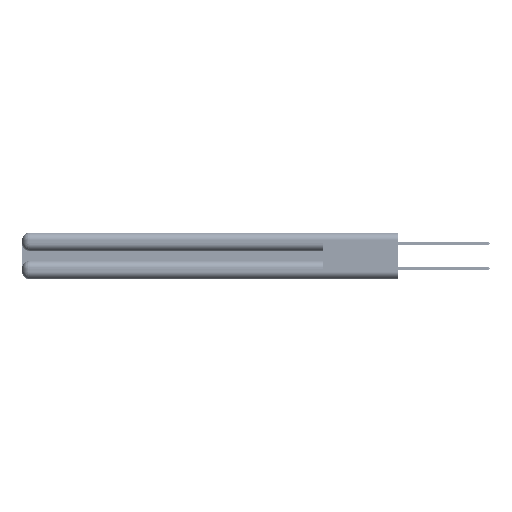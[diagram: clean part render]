
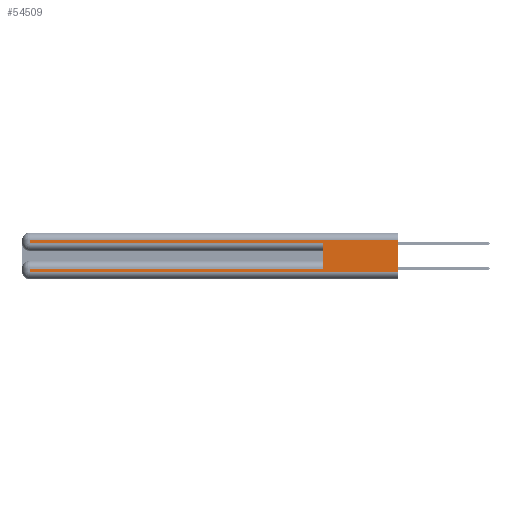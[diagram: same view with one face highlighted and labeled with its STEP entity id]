
A CAD part, left-side view. The second image highlights one B-rep face of the part: STEP entity #54509.
In plain terms, the highlighted planar face has unit normal (-1, 0, 0).
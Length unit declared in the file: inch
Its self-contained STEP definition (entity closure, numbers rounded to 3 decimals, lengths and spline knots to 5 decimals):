
#398 = VECTOR ( 'NONE', #5086, 39.37008 ) ;
#578 = VERTEX_POINT ( 'NONE', #2584 ) ;
#615 = CARTESIAN_POINT ( 'NONE',  ( 0., 0., 0.06 ) ) ;
#1155 = ORIENTED_EDGE ( 'NONE', *, *, #53234, .T. ) ;
#1574 = VECTOR ( 'NONE', #17906, 39.37008 ) ;
#2584 = CARTESIAN_POINT ( 'NONE',  ( 0., 0.6, 0.085 ) ) ;
#5034 = CARTESIAN_POINT ( 'NONE',  ( 0., 2.94, 0.37 ) ) ;
#5086 = DIRECTION ( 'NONE',  ( 0., 0., -1. ) ) ;
#5473 = VERTEX_POINT ( 'NONE', #21969 ) ;
#5600 = FACE_OUTER_BOUND ( 'NONE', #11197, .T. ) ;
#6402 = LINE ( 'NONE', #31272, #38980 ) ;
#7003 = ORIENTED_EDGE ( 'NONE', *, *, #23486, .F. ) ;
#7618 = CARTESIAN_POINT ( 'NONE',  ( 0., 0., 0.06 ) ) ;
#8330 = VECTOR ( 'NONE', #22632, 39.37008 ) ;
#8493 = CARTESIAN_POINT ( 'NONE',  ( 0., 0., 0.37 ) ) ;
#9296 = DIRECTION ( 'NONE',  ( 0., 0., -1. ) ) ;
#9761 = LINE ( 'NONE', #21096, #29712 ) ;
#10729 = CARTESIAN_POINT ( 'NONE',  ( 0., 2.94, 0.31 ) ) ;
#11197 = EDGE_LOOP ( 'NONE', ( #7003, #38644, #1155, #52044, #32829, #33176, #42025, #19998 ) ) ;
#12779 = DIRECTION ( 'NONE',  ( 0., 0., -1. ) ) ;
#12935 = VERTEX_POINT ( 'NONE', #10729 ) ;
#13240 = CARTESIAN_POINT ( 'NONE',  ( 0., 0.6, 0.285 ) ) ;
#14727 = VECTOR ( 'NONE', #20359, 39.37008 ) ;
#17906 = DIRECTION ( 'NONE',  ( 0., 0., 1. ) ) ;
#18385 = EDGE_CURVE ( 'NONE', #5473, #44259, #18519, .T. ) ;
#18519 = LINE ( 'NONE', #7618, #28480 ) ;
#19662 = LINE ( 'NONE', #52302, #8330 ) ;
#19998 = ORIENTED_EDGE ( 'NONE', *, *, #18385, .T. ) ;
#20359 = DIRECTION ( 'NONE',  ( 0., 0., -1. ) ) ;
#21096 = CARTESIAN_POINT ( 'NONE',  ( 0., 0., 0.285 ) ) ;
#21969 = CARTESIAN_POINT ( 'NONE',  ( 0., 2.94, 0.06 ) ) ;
#22632 = DIRECTION ( 'NONE',  ( 0., 1., 0. ) ) ;
#23486 = EDGE_CURVE ( 'NONE', #52811, #44259, #48574, .T. ) ;
#25427 = PLANE ( 'NONE',  #37599 ) ;
#26331 = EDGE_CURVE ( 'NONE', #32562, #36305, #9761, .T. ) ;
#27882 = EDGE_CURVE ( 'NONE', #52811, #12935, #19662, .T. ) ;
#28480 = VECTOR ( 'NONE', #37346, 39.37008 ) ;
#28507 = EDGE_CURVE ( 'NONE', #578, #36305, #35522, .T. ) ;
#29712 = VECTOR ( 'NONE', #46698, 39.37008 ) ;
#31272 = CARTESIAN_POINT ( 'NONE',  ( 0., 0., 0.085 ) ) ;
#31387 = VECTOR ( 'NONE', #9296, 39.37008 ) ;
#32481 = CARTESIAN_POINT ( 'NONE',  ( 0., 2.94, 0.285 ) ) ;
#32562 = VERTEX_POINT ( 'NONE', #32481 ) ;
#32829 = ORIENTED_EDGE ( 'NONE', *, *, #28507, .F. ) ;
#33176 = ORIENTED_EDGE ( 'NONE', *, *, #53359, .T. ) ;
#34354 = LINE ( 'NONE', #34819, #398 ) ;
#34819 = CARTESIAN_POINT ( 'NONE',  ( 0., 2.94, 0.37 ) ) ;
#35522 = LINE ( 'NONE', #47583, #1574 ) ;
#35553 = DIRECTION ( 'NONE',  ( 0., 1., 0. ) ) ;
#35851 = VERTEX_POINT ( 'NONE', #52831 ) ;
#36305 = VERTEX_POINT ( 'NONE', #13240 ) ;
#37346 = DIRECTION ( 'NONE',  ( 0., -1., 0. ) ) ;
#37599 = AXIS2_PLACEMENT_3D ( 'NONE', #8493, #38223, #12779 ) ;
#38223 = DIRECTION ( 'NONE',  ( 1., 0., 0. ) ) ;
#38644 = ORIENTED_EDGE ( 'NONE', *, *, #27882, .T. ) ;
#38980 = VECTOR ( 'NONE', #35553, 39.37008 ) ;
#40806 = CARTESIAN_POINT ( 'NONE',  ( 0., 0., 0.31 ) ) ;
#41697 = CARTESIAN_POINT ( 'NONE',  ( 0., 0., 0.37 ) ) ;
#42025 = ORIENTED_EDGE ( 'NONE', *, *, #49187, .T. ) ;
#44033 = LINE ( 'NONE', #5034, #31387 ) ;
#44259 = VERTEX_POINT ( 'NONE', #615 ) ;
#46698 = DIRECTION ( 'NONE',  ( 0., -1., 0. ) ) ;
#47583 = CARTESIAN_POINT ( 'NONE',  ( 0., 0.6, 0.145 ) ) ;
#48574 = LINE ( 'NONE', #41697, #14727 ) ;
#49187 = EDGE_CURVE ( 'NONE', #35851, #5473, #44033, .T. ) ;
#52044 = ORIENTED_EDGE ( 'NONE', *, *, #26331, .T. ) ;
#52302 = CARTESIAN_POINT ( 'NONE',  ( 0., 0., 0.31 ) ) ;
#52811 = VERTEX_POINT ( 'NONE', #40806 ) ;
#52831 = CARTESIAN_POINT ( 'NONE',  ( 0., 2.94, 0.085 ) ) ;
#53234 = EDGE_CURVE ( 'NONE', #12935, #32562, #34354, .T. ) ;
#53359 = EDGE_CURVE ( 'NONE', #578, #35851, #6402, .T. ) ;
#54509 = ADVANCED_FACE ( 'NONE', ( #5600 ), #25427, .F. ) ;
